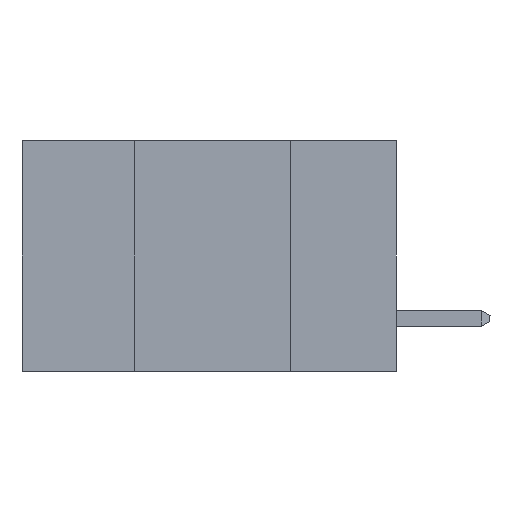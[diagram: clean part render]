
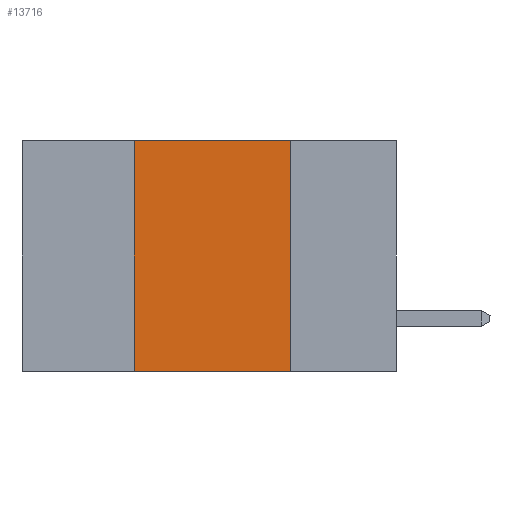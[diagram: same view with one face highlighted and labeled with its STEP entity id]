
A CAD part, left-side view. The second image highlights one B-rep face of the part: STEP entity #13716.
In plain terms, the highlighted planar face has unit normal (-1, 0, 0).
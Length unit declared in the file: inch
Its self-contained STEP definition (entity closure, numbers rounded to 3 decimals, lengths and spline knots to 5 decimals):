
#512 = ORIENTED_EDGE ( 'NONE', *, *, #5949, .T. ) ;
#688 = DIRECTION ( 'NONE',  ( 0., -1., 0. ) ) ;
#1780 = CARTESIAN_POINT ( 'NONE',  ( 0., 0.17, -0.37 ) ) ;
#1988 = DIRECTION ( 'NONE',  ( 0., 0., 1. ) ) ;
#2118 = CARTESIAN_POINT ( 'NONE',  ( 0., 0.42, -0.37 ) ) ;
#3493 = AXIS2_PLACEMENT_3D ( 'NONE', #6860, #17714, #8421 ) ;
#5071 = DIRECTION ( 'NONE',  ( 0., 0., -1. ) ) ;
#5738 = VECTOR ( 'NONE', #5071, 39.37008 ) ;
#5949 = EDGE_CURVE ( 'NONE', #16221, #12238, #6032, .T. ) ;
#6032 = LINE ( 'NONE', #17001, #13827 ) ;
#6484 = VERTEX_POINT ( 'NONE', #14434 ) ;
#6860 = CARTESIAN_POINT ( 'NONE',  ( 0., 0.6, 0. ) ) ;
#7200 = VERTEX_POINT ( 'NONE', #11068 ) ;
#7733 = LINE ( 'NONE', #2118, #11351 ) ;
#8073 = EDGE_CURVE ( 'NONE', #16221, #7200, #7733, .T. ) ;
#8421 = DIRECTION ( 'NONE',  ( 0., 0., -1. ) ) ;
#9448 = LINE ( 'NONE', #14427, #5738 ) ;
#10938 = CARTESIAN_POINT ( 'NONE',  ( 0., 0.42, -0.37 ) ) ;
#11068 = CARTESIAN_POINT ( 'NONE',  ( 0., 0.42, 0. ) ) ;
#11184 = EDGE_CURVE ( 'NONE', #7200, #6484, #19157, .T. ) ;
#11351 = VECTOR ( 'NONE', #1988, 39.37008 ) ;
#12238 = VERTEX_POINT ( 'NONE', #1780 ) ;
#13353 = FACE_OUTER_BOUND ( 'NONE', #14765, .T. ) ;
#13666 = DIRECTION ( 'NONE',  ( 0., -1., 0. ) ) ;
#13716 = ADVANCED_FACE ( 'NONE', ( #13353 ), #16127, .F. ) ;
#13798 = ORIENTED_EDGE ( 'NONE', *, *, #14301, .F. ) ;
#13827 = VECTOR ( 'NONE', #688, 39.37008 ) ;
#13836 = CARTESIAN_POINT ( 'NONE',  ( 0., 0.6, 0. ) ) ;
#14301 = EDGE_CURVE ( 'NONE', #6484, #12238, #9448, .T. ) ;
#14427 = CARTESIAN_POINT ( 'NONE',  ( 0., 0.17, -0.37 ) ) ;
#14434 = CARTESIAN_POINT ( 'NONE',  ( 0., 0.17, 0. ) ) ;
#14765 = EDGE_LOOP ( 'NONE', ( #13798, #15034, #16335, #512 ) ) ;
#15034 = ORIENTED_EDGE ( 'NONE', *, *, #11184, .F. ) ;
#16127 = PLANE ( 'NONE',  #3493 ) ;
#16221 = VERTEX_POINT ( 'NONE', #10938 ) ;
#16335 = ORIENTED_EDGE ( 'NONE', *, *, #8073, .F. ) ;
#17001 = CARTESIAN_POINT ( 'NONE',  ( 0., 0.6, -0.37 ) ) ;
#17714 = DIRECTION ( 'NONE',  ( 1., 0., 0. ) ) ;
#18275 = VECTOR ( 'NONE', #13666, 39.37008 ) ;
#19157 = LINE ( 'NONE', #13836, #18275 ) ;
